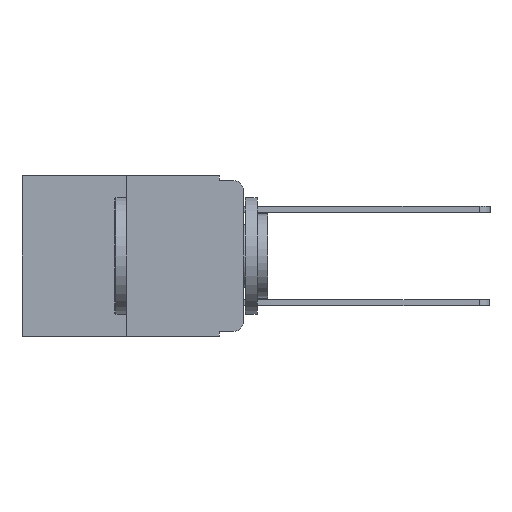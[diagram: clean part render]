
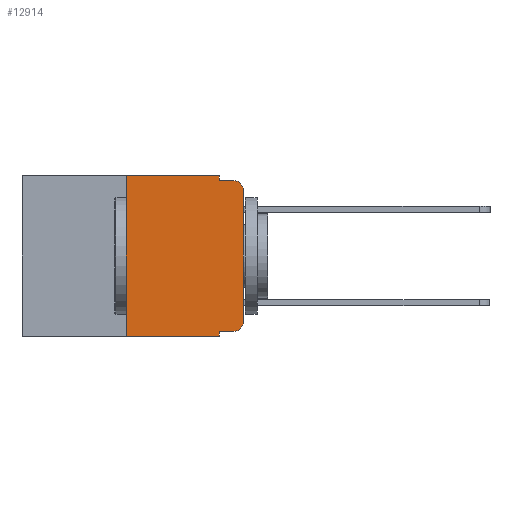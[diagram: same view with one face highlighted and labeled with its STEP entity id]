
A CAD part, left-side view. The second image highlights one B-rep face of the part: STEP entity #12914.
In plain terms, the highlighted planar face has unit normal (-1, 0, 0).
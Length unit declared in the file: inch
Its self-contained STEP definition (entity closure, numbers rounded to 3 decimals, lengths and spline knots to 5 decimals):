
#76 = ORIENTED_EDGE ( 'NONE', *, *, #8962, .T. ) ;
#260 = CARTESIAN_POINT ( 'NONE',  ( 0., 0.051, -0.343 ) ) ;
#306 = ORIENTED_EDGE ( 'NONE', *, *, #12036, .T. ) ;
#343 = ORIENTED_EDGE ( 'NONE', *, *, #1551, .F. ) ;
#507 = CARTESIAN_POINT ( 'NONE',  ( 0., 0.051, 0. ) ) ;
#546 = CARTESIAN_POINT ( 'NONE',  ( 0., 0.02, -0.03 ) ) ;
#707 = CARTESIAN_POINT ( 'NONE',  ( 0., 0.051, -0.01 ) ) ;
#738 = PLANE ( 'NONE',  #8275 ) ;
#1042 = DIRECTION ( 'NONE',  ( 0., -1., 0. ) ) ;
#1210 = ORIENTED_EDGE ( 'NONE', *, *, #4839, .F. ) ;
#1317 = ORIENTED_EDGE ( 'NONE', *, *, #8472, .T. ) ;
#1337 = LINE ( 'NONE', #2054, #1721 ) ;
#1532 = VERTEX_POINT ( 'NONE', #8799 ) ;
#1551 = EDGE_CURVE ( 'NONE', #6343, #1571, #11119, .T. ) ;
#1571 = VERTEX_POINT ( 'NONE', #2014 ) ;
#1721 = VECTOR ( 'NONE', #11809, 39.37008 ) ;
#1805 = ORIENTED_EDGE ( 'NONE', *, *, #6366, .F. ) ;
#1851 = DIRECTION ( 'NONE',  ( 0., 0., -1. ) ) ;
#1865 = ORIENTED_EDGE ( 'NONE', *, *, #13400, .T. ) ;
#2014 = CARTESIAN_POINT ( 'NONE',  ( 0., 0.02, -0.01 ) ) ;
#2054 = CARTESIAN_POINT ( 'NONE',  ( 0., 0.473, -0.343 ) ) ;
#2383 = CARTESIAN_POINT ( 'NONE',  ( 0., 0.02, -0.333 ) ) ;
#2750 = CARTESIAN_POINT ( 'NONE',  ( 0., 0.25, 0. ) ) ;
#2997 = CIRCLE ( 'NONE', #12881, 0.02 ) ;
#3524 = DIRECTION ( 'NONE',  ( 0., -1., 0. ) ) ;
#3771 = ORIENTED_EDGE ( 'NONE', *, *, #5603, .F. ) ;
#3869 = CARTESIAN_POINT ( 'NONE',  ( 0., 0.02, -0.313 ) ) ;
#4373 = DIRECTION ( 'NONE',  ( 0., 0., 1. ) ) ;
#4628 = DIRECTION ( 'NONE',  ( 0., -1., 0. ) ) ;
#4716 = VECTOR ( 'NONE', #9974, 39.37008 ) ;
#4827 = AXIS2_PLACEMENT_3D ( 'NONE', #546, #8666, #1851 ) ;
#4839 = EDGE_CURVE ( 'NONE', #5203, #6343, #10823, .T. ) ;
#5110 = DIRECTION ( 'NONE',  ( 0., 0., -1. ) ) ;
#5203 = VERTEX_POINT ( 'NONE', #507 ) ;
#5344 = VECTOR ( 'NONE', #4628, 39.37008 ) ;
#5603 = EDGE_CURVE ( 'NONE', #1532, #10460, #10344, .T. ) ;
#5634 = VECTOR ( 'NONE', #1042, 39.37008 ) ;
#5660 = DIRECTION ( 'NONE',  ( 0., 0., -1. ) ) ;
#5756 = VECTOR ( 'NONE', #3524, 39.37008 ) ;
#5891 = VERTEX_POINT ( 'NONE', #9071 ) ;
#6343 = VERTEX_POINT ( 'NONE', #12929 ) ;
#6366 = EDGE_CURVE ( 'NONE', #5891, #9925, #13296, .T. ) ;
#6503 = VERTEX_POINT ( 'NONE', #10145 ) ;
#6728 = CARTESIAN_POINT ( 'NONE',  ( 0., 0.473, 0. ) ) ;
#7598 = EDGE_CURVE ( 'NONE', #10460, #5203, #11214, .T. ) ;
#8022 = CARTESIAN_POINT ( 'NONE',  ( 0., 0.473, 0. ) ) ;
#8159 = VECTOR ( 'NONE', #9087, 39.37008 ) ;
#8275 = AXIS2_PLACEMENT_3D ( 'NONE', #6728, #11793, #5660 ) ;
#8472 = EDGE_CURVE ( 'NONE', #5891, #13081, #10571, .T. ) ;
#8666 = DIRECTION ( 'NONE',  ( -1., 0., 0. ) ) ;
#8799 = CARTESIAN_POINT ( 'NONE',  ( 0., 0.25, -0.343 ) ) ;
#8962 = EDGE_CURVE ( 'NONE', #1532, #9925, #1337, .T. ) ;
#9071 = CARTESIAN_POINT ( 'NONE',  ( 0., 0.051, -0.333 ) ) ;
#9087 = DIRECTION ( 'NONE',  ( 0., 0., -1. ) ) ;
#9103 = ORIENTED_EDGE ( 'NONE', *, *, #11365, .T. ) ;
#9130 = EDGE_LOOP ( 'NONE', ( #306, #1865, #343, #1210, #11581, #3771, #76, #1805, #1317, #9103 ) ) ;
#9925 = VERTEX_POINT ( 'NONE', #260 ) ;
#9974 = DIRECTION ( 'NONE',  ( 0., 0., -1. ) ) ;
#10145 = CARTESIAN_POINT ( 'NONE',  ( 0., 0., -0.313 ) ) ;
#10344 = LINE ( 'NONE', #10730, #10651 ) ;
#10460 = VERTEX_POINT ( 'NONE', #2750 ) ;
#10488 = VECTOR ( 'NONE', #12286, 39.37008 ) ;
#10571 = LINE ( 'NONE', #10931, #5344 ) ;
#10651 = VECTOR ( 'NONE', #4373, 39.37008 ) ;
#10730 = CARTESIAN_POINT ( 'NONE',  ( 0., 0.25, 0. ) ) ;
#10823 = LINE ( 'NONE', #12009, #8159 ) ;
#10931 = CARTESIAN_POINT ( 'NONE',  ( 0., 0.051, -0.333 ) ) ;
#11119 = LINE ( 'NONE', #707, #5634 ) ;
#11214 = LINE ( 'NONE', #8022, #5756 ) ;
#11316 = DIRECTION ( 'NONE',  ( -1., 0., 0. ) ) ;
#11365 = EDGE_CURVE ( 'NONE', #13081, #6503, #2997, .T. ) ;
#11581 = ORIENTED_EDGE ( 'NONE', *, *, #7598, .F. ) ;
#11793 = DIRECTION ( 'NONE',  ( 1., 0., 0. ) ) ;
#11809 = DIRECTION ( 'NONE',  ( 0., -1., 0. ) ) ;
#12009 = CARTESIAN_POINT ( 'NONE',  ( 0., 0.051, 0. ) ) ;
#12036 = EDGE_CURVE ( 'NONE', #6503, #12774, #13437, .T. ) ;
#12286 = DIRECTION ( 'NONE',  ( 0., 0., 1. ) ) ;
#12437 = CIRCLE ( 'NONE', #4827, 0.02 ) ;
#12541 = CARTESIAN_POINT ( 'NONE',  ( 0., 0., -0.03 ) ) ;
#12774 = VERTEX_POINT ( 'NONE', #12541 ) ;
#12782 = FACE_OUTER_BOUND ( 'NONE', #9130, .T. ) ;
#12881 = AXIS2_PLACEMENT_3D ( 'NONE', #3869, #11316, #5110 ) ;
#12914 = ADVANCED_FACE ( 'NONE', ( #12782 ), #738, .F. ) ;
#12929 = CARTESIAN_POINT ( 'NONE',  ( 0., 0.051, -0.01 ) ) ;
#13081 = VERTEX_POINT ( 'NONE', #2383 ) ;
#13271 = CARTESIAN_POINT ( 'NONE',  ( 0., 0., 0. ) ) ;
#13296 = LINE ( 'NONE', #13945, #4716 ) ;
#13400 = EDGE_CURVE ( 'NONE', #12774, #1571, #12437, .T. ) ;
#13437 = LINE ( 'NONE', #13271, #10488 ) ;
#13945 = CARTESIAN_POINT ( 'NONE',  ( 0., 0.051, 0. ) ) ;
